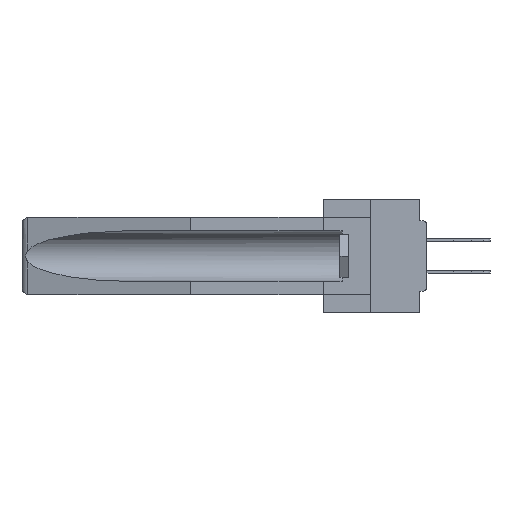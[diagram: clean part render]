
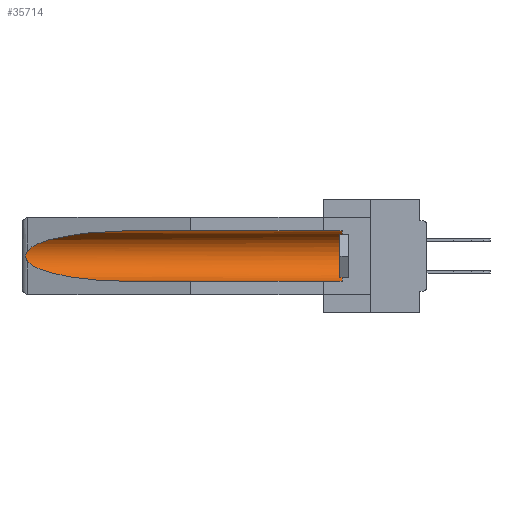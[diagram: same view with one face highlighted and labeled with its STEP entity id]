
A CAD part, left-side view. The second image highlights one B-rep face of the part: STEP entity #35714.
In plain terms, the highlighted cylindrical face has radius 2.857 mm (diameter 5.715 mm), a partial arc.
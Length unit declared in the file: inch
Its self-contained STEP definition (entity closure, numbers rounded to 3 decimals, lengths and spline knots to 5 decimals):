
#213 = DIRECTION ( 'NONE',  ( 0., 0., 1. ) ) ;
#296 = ORIENTED_EDGE ( 'NONE', *, *, #10602, .F. ) ;
#569 = CARTESIAN_POINT ( 'NONE',  ( 0.26537, 1.52718, -0.19328 ) ) ;
#1261 = VERTEX_POINT ( 'NONE', #25763 ) ;
#2896 = ORIENTED_EDGE ( 'NONE', *, *, #33409, .T. ) ;
#3194 = CARTESIAN_POINT ( 'NONE',  ( 0.26597, 1.52961, -0.15275 ) ) ;
#6021 =( BOUNDED_CURVE ( )  B_SPLINE_CURVE ( 3, ( #28449, #28720, #11843, #35414 ),
 .UNSPECIFIED., .F., .T. ) 
 B_SPLINE_CURVE_WITH_KNOTS ( ( 4, 4 ),
 ( 0.1948, 1.5708 ),
 .UNSPECIFIED. ) 
 CURVE ( )  GEOMETRIC_REPRESENTATION_ITEM ( )  RATIONAL_B_SPLINE_CURVE ( ( 1., 0.848, 0.848, 1. ) ) 
 REPRESENTATION_ITEM ( '' )  );
#7804 = CARTESIAN_POINT ( 'NONE',  ( 0.2673, 1.5327, -0.16383 ) ) ;
#8519 = ORIENTED_EDGE ( 'NONE', *, *, #24466, .T. ) ;
#9708 = VERTEX_POINT ( 'NONE', #40364 ) ;
#9967 = B_SPLINE_CURVE_WITH_KNOTS ( 'NONE', 3,
 ( #39161, #3194, #20630, #7804, #37378, #10994, #20925, #31086, #40735, #569 ),
 .UNSPECIFIED., .F., .F.,
 ( 4, 2, 2, 2, 4 ),
 ( 0., 0.00029, 0.00058, 0.00087, 0.00117 ),
 .UNSPECIFIED. ) ;
#10602 = EDGE_CURVE ( 'NONE', #1261, #9708, #35351, .T. ) ;
#10994 = CARTESIAN_POINT ( 'NONE',  ( 0.2675, 1.53308, -0.17534 ) ) ;
#11548 = CARTESIAN_POINT ( 'NONE',  ( 0.26537, 1.52718, -0.14972 ) ) ;
#11843 = CARTESIAN_POINT ( 'NONE',  ( 0.21114, 1.30732, -0.284 ) ) ;
#12627 = VERTEX_POINT ( 'NONE', #19340 ) ;
#12698 = CARTESIAN_POINT ( 'NONE',  ( 0.25451, 1.48313, -0.09465 ) ) ;
#13639 = LINE ( 'NONE', #22263, #35534 ) ;
#14534 = VECTOR ( 'NONE', #37189, 39.37008 ) ;
#15628 = CARTESIAN_POINT ( 'NONE',  ( 0.26537, 1.52718, -0.14972 ) ) ;
#16383 = CARTESIAN_POINT ( 'NONE',  ( 0.155, -0.30754, -0.284 ) ) ;
#16436 = EDGE_CURVE ( 'NONE', #12627, #22657, #29206, .T. ) ;
#16721 = CARTESIAN_POINT ( 'NONE',  ( 0.26537, 1.52718, -0.19328 ) ) ;
#17900 = DIRECTION ( 'NONE',  ( 0., 1., 0. ) ) ;
#19088 = ORIENTED_EDGE ( 'NONE', *, *, #21367, .T. ) ;
#19340 = CARTESIAN_POINT ( 'NONE',  ( 0.155, 1.07973, -0.059 ) ) ;
#19857 = CARTESIAN_POINT ( 'NONE',  ( 0.155, 0.126, -0.1715 ) ) ;
#20630 = CARTESIAN_POINT ( 'NONE',  ( 0.26654, 1.53092, -0.15636 ) ) ;
#20925 = CARTESIAN_POINT ( 'NONE',  ( 0.2673, 1.53269, -0.17917 ) ) ;
#21367 = EDGE_CURVE ( 'NONE', #1261, #42581, #41841, .T. ) ;
#21897 = CYLINDRICAL_SURFACE ( 'NONE', #40573, 0.1125 ) ;
#22263 = CARTESIAN_POINT ( 'NONE',  ( 0.155, -0.30754, -0.059 ) ) ;
#22657 = VERTEX_POINT ( 'NONE', #11548 ) ;
#24186 = ORIENTED_EDGE ( 'NONE', *, *, #16436, .T. ) ;
#24466 = EDGE_CURVE ( 'NONE', #42581, #12627, #13639, .T. ) ;
#24969 = VERTEX_POINT ( 'NONE', #16721 ) ;
#25423 = AXIS2_PLACEMENT_3D ( 'NONE', #19857, #36873, #213 ) ;
#25763 = CARTESIAN_POINT ( 'NONE',  ( 0.155, 0.126, -0.284 ) ) ;
#25837 = CARTESIAN_POINT ( 'NONE',  ( 0.155, 1.07973, -0.059 ) ) ;
#25869 = EDGE_CURVE ( 'NONE', #24969, #9708, #6021, .T. ) ;
#27783 = DIRECTION ( 'NONE',  ( 0., 0., 1. ) ) ;
#28174 = ORIENTED_EDGE ( 'NONE', *, *, #25869, .T. ) ;
#28449 = CARTESIAN_POINT ( 'NONE',  ( 0.26537, 1.52718, -0.19328 ) ) ;
#28720 = CARTESIAN_POINT ( 'NONE',  ( 0.25451, 1.48313, -0.24835 ) ) ;
#29206 =( BOUNDED_CURVE ( )  B_SPLINE_CURVE ( 3, ( #25837, #42183, #12698, #15628 ),
 .UNSPECIFIED., .F., .T. ) 
 B_SPLINE_CURVE_WITH_KNOTS ( ( 4, 4 ),
 ( 4.71239, 6.08839 ),
 .UNSPECIFIED. ) 
 CURVE ( )  GEOMETRIC_REPRESENTATION_ITEM ( )  RATIONAL_B_SPLINE_CURVE ( ( 1., 0.848, 0.848, 1. ) ) 
 REPRESENTATION_ITEM ( '' )  );
#30720 = FACE_OUTER_BOUND ( 'NONE', #41295, .T. ) ;
#31086 = CARTESIAN_POINT ( 'NONE',  ( 0.26655, 1.53094, -0.18657 ) ) ;
#33409 = EDGE_CURVE ( 'NONE', #22657, #24969, #9967, .T. ) ;
#34318 = CARTESIAN_POINT ( 'NONE',  ( 0.155, -0.30754, -0.1715 ) ) ;
#35351 = LINE ( 'NONE', #16383, #14534 ) ;
#35414 = CARTESIAN_POINT ( 'NONE',  ( 0.155, 1.07973, -0.284 ) ) ;
#35534 = VECTOR ( 'NONE', #39009, 39.37008 ) ;
#35714 = ADVANCED_FACE ( 'NONE', ( #30720 ), #21897, .F. ) ;
#36873 = DIRECTION ( 'NONE',  ( 0., -1., 0. ) ) ;
#37189 = DIRECTION ( 'NONE',  ( 0., 1., 0. ) ) ;
#37378 = CARTESIAN_POINT ( 'NONE',  ( 0.2675, 1.53308, -0.16763 ) ) ;
#38671 = CARTESIAN_POINT ( 'NONE',  ( 0.155, 0.126, -0.059 ) ) ;
#39009 = DIRECTION ( 'NONE',  ( 0., 1., 0. ) ) ;
#39161 = CARTESIAN_POINT ( 'NONE',  ( 0.26537, 1.52718, -0.14972 ) ) ;
#40364 = CARTESIAN_POINT ( 'NONE',  ( 0.155, 1.07973, -0.284 ) ) ;
#40573 = AXIS2_PLACEMENT_3D ( 'NONE', #34318, #17900, #27783 ) ;
#40735 = CARTESIAN_POINT ( 'NONE',  ( 0.26597, 1.5296, -0.19026 ) ) ;
#41295 = EDGE_LOOP ( 'NONE', ( #24186, #2896, #28174, #296, #19088, #8519 ) ) ;
#41841 = CIRCLE ( 'NONE', #25423, 0.1125 ) ;
#42183 = CARTESIAN_POINT ( 'NONE',  ( 0.21114, 1.30732, -0.059 ) ) ;
#42581 = VERTEX_POINT ( 'NONE', #38671 ) ;
